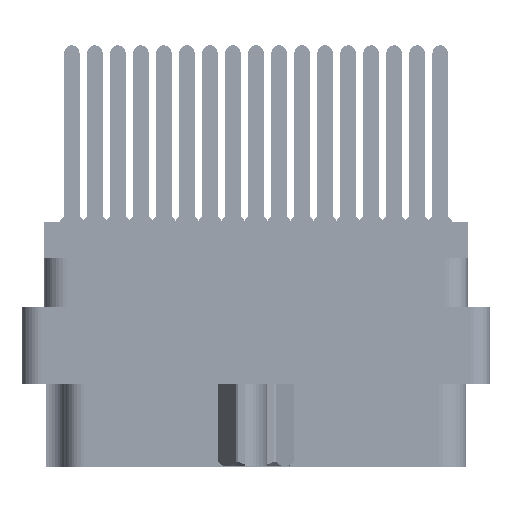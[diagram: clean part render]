
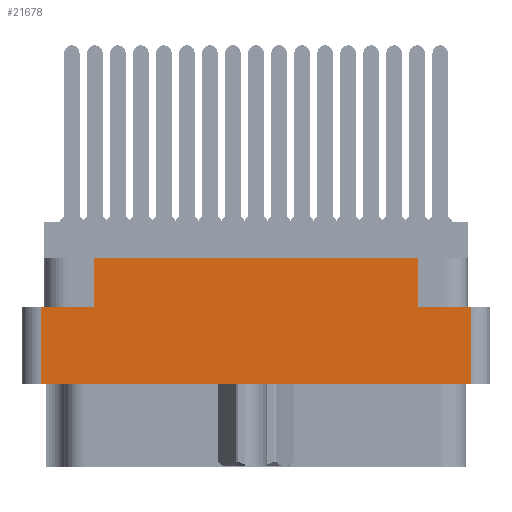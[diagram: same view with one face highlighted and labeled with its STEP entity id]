
A CAD part, left-side view. The second image highlights one B-rep face of the part: STEP entity #21678.
In plain terms, the highlighted planar face has unit normal (-1, 0, 0).
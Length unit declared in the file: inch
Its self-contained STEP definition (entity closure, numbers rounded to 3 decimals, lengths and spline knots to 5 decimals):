
#1694 = VERTEX_POINT ( 'NONE', #88443 ) ;
#5329 = VERTEX_POINT ( 'NONE', #38738 ) ;
#6908 = DIRECTION ( 'NONE',  ( 0., 0., 1. ) ) ;
#8547 = ORIENTED_EDGE ( 'NONE', *, *, #50683, .T. ) ;
#10154 = VECTOR ( 'NONE', #6908, 39.37008 ) ;
#12937 = LINE ( 'NONE', #61610, #65690 ) ;
#13041 = CARTESIAN_POINT ( 'NONE',  ( -1.375, -0.5285, -0.277 ) ) ;
#13398 = VERTEX_POINT ( 'NONE', #13041 ) ;
#13844 = ORIENTED_EDGE ( 'NONE', *, *, #27119, .F. ) ;
#15367 = ORIENTED_EDGE ( 'NONE', *, *, #51684, .F. ) ;
#17056 = DIRECTION ( 'NONE',  ( 0., 0., 1. ) ) ;
#18849 = LINE ( 'NONE', #34122, #97717 ) ;
#21678 = ADVANCED_FACE ( 'NONE', ( #80059 ), #32230, .T. ) ;
#21915 = DIRECTION ( 'NONE',  ( 0., 1., 0. ) ) ;
#23667 = DIRECTION ( 'NONE',  ( 0., -1., 0. ) ) ;
#27119 = EDGE_CURVE ( 'NONE', #5329, #86753, #12937, .T. ) ;
#29468 = LINE ( 'NONE', #101995, #53408 ) ;
#30060 = LINE ( 'NONE', #49225, #71412 ) ;
#30256 = LINE ( 'NONE', #98602, #91565 ) ;
#32230 = PLANE ( 'NONE',  #45560 ) ;
#33475 = LINE ( 'NONE', #103230, #103509 ) ;
#34122 = CARTESIAN_POINT ( 'NONE',  ( -1.375, -0.7005, -0.798 ) ) ;
#35117 = CARTESIAN_POINT ( 'NONE',  ( -1.375, 0.7005, -0.277 ) ) ;
#38738 = CARTESIAN_POINT ( 'NONE',  ( -1.375, -0.7005, -0.529 ) ) ;
#42086 = EDGE_CURVE ( 'NONE', #13398, #70822, #95922, .T. ) ;
#45560 = AXIS2_PLACEMENT_3D ( 'NONE', #64121, #48077, #17056 ) ;
#45898 = CARTESIAN_POINT ( 'NONE',  ( -1.375, 0.5285, -0.277 ) ) ;
#48077 = DIRECTION ( 'NONE',  ( -1., 0., 0. ) ) ;
#49225 = CARTESIAN_POINT ( 'NONE',  ( -1.375, 0., -0.277 ) ) ;
#50251 = VERTEX_POINT ( 'NONE', #35117 ) ;
#50683 = EDGE_CURVE ( 'NONE', #50251, #86753, #33475, .T. ) ;
#50856 = DIRECTION ( 'NONE',  ( 0., -1., 0. ) ) ;
#51684 = EDGE_CURVE ( 'NONE', #93047, #1694, #29468, .T. ) ;
#52939 = LINE ( 'NONE', #55019, #10154 ) ;
#53408 = VECTOR ( 'NONE', #83466, 39.37008 ) ;
#55019 = CARTESIAN_POINT ( 'NONE',  ( -1.375, -0.5285, -0.277 ) ) ;
#61610 = CARTESIAN_POINT ( 'NONE',  ( -1.375, 0., -0.529 ) ) ;
#62552 = ORIENTED_EDGE ( 'NONE', *, *, #42086, .F. ) ;
#64121 = CARTESIAN_POINT ( 'NONE',  ( -1.375, -0.7625, -0.798 ) ) ;
#65292 = ORIENTED_EDGE ( 'NONE', *, *, #79739, .F. ) ;
#65690 = VECTOR ( 'NONE', #21915, 39.37008 ) ;
#70438 = CARTESIAN_POINT ( 'NONE',  ( -1.375, -0.7005, -0.277 ) ) ;
#70697 = CARTESIAN_POINT ( 'NONE',  ( -1.375, 0., -0.277 ) ) ;
#70822 = VERTEX_POINT ( 'NONE', #70438 ) ;
#71412 = VECTOR ( 'NONE', #80571, 39.37008 ) ;
#74724 = DIRECTION ( 'NONE',  ( 0., 0., 1. ) ) ;
#74811 = CARTESIAN_POINT ( 'NONE',  ( -1.375, -0.5285, -0.117 ) ) ;
#79563 = ORIENTED_EDGE ( 'NONE', *, *, #100666, .T. ) ;
#79739 = EDGE_CURVE ( 'NONE', #50251, #93047, #30060, .T. ) ;
#80059 = FACE_OUTER_BOUND ( 'NONE', #93182, .T. ) ;
#80571 = DIRECTION ( 'NONE',  ( 0., -1., 0. ) ) ;
#81598 = ORIENTED_EDGE ( 'NONE', *, *, #83470, .T. ) ;
#83145 = VERTEX_POINT ( 'NONE', #74811 ) ;
#83466 = DIRECTION ( 'NONE',  ( 0., 0., 1. ) ) ;
#83470 = EDGE_CURVE ( 'NONE', #5329, #70822, #18849, .T. ) ;
#84670 = VECTOR ( 'NONE', #23667, 39.37008 ) ;
#84845 = ORIENTED_EDGE ( 'NONE', *, *, #91015, .F. ) ;
#86753 = VERTEX_POINT ( 'NONE', #98715 ) ;
#88443 = CARTESIAN_POINT ( 'NONE',  ( -1.375, 0.5285, -0.117 ) ) ;
#91015 = EDGE_CURVE ( 'NONE', #1694, #83145, #30256, .T. ) ;
#91565 = VECTOR ( 'NONE', #50856, 39.37008 ) ;
#93047 = VERTEX_POINT ( 'NONE', #45898 ) ;
#93182 = EDGE_LOOP ( 'NONE', ( #65292, #8547, #13844, #81598, #62552, #79563, #84845, #15367 ) ) ;
#95231 = DIRECTION ( 'NONE',  ( 0., 0., -1. ) ) ;
#95922 = LINE ( 'NONE', #70697, #84670 ) ;
#97717 = VECTOR ( 'NONE', #74724, 39.37008 ) ;
#98602 = CARTESIAN_POINT ( 'NONE',  ( -1.375, 0.7625, -0.117 ) ) ;
#98715 = CARTESIAN_POINT ( 'NONE',  ( -1.375, 0.7005, -0.529 ) ) ;
#100666 = EDGE_CURVE ( 'NONE', #13398, #83145, #52939, .T. ) ;
#101995 = CARTESIAN_POINT ( 'NONE',  ( -1.375, 0.5285, -0.277 ) ) ;
#103230 = CARTESIAN_POINT ( 'NONE',  ( -1.375, 0.7005, -0.798 ) ) ;
#103509 = VECTOR ( 'NONE', #95231, 39.37008 ) ;
